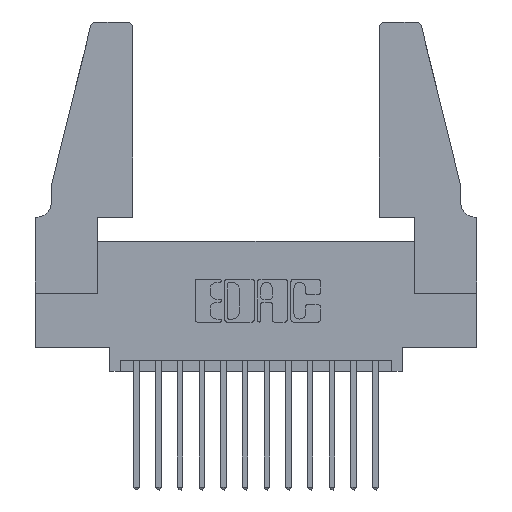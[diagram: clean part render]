
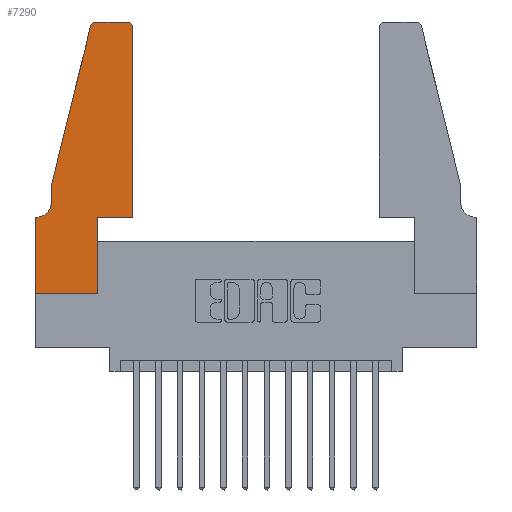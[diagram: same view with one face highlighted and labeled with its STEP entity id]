
A CAD part, top view. The second image highlights one B-rep face of the part: STEP entity #7290.
In plain terms, the highlighted planar face has unit normal (0, 0, 1).
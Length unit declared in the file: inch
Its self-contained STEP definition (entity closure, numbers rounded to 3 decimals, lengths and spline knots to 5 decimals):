
#84 = VECTOR ( 'NONE', #13092, 39.37008 ) ;
#192 = DIRECTION ( 'NONE',  ( 0., 0., 1. ) ) ;
#492 = CARTESIAN_POINT ( 'NONE',  ( 0.0755, 0.42, 0.37 ) ) ;
#546 = CARTESIAN_POINT ( 'NONE',  ( 0., 0., 0.37 ) ) ;
#605 = CARTESIAN_POINT ( 'NONE',  ( 0.0755, 0.5, 0.37 ) ) ;
#638 = AXIS2_PLACEMENT_3D ( 'NONE', #14858, #8767, #1571 ) ;
#672 = DIRECTION ( 'NONE',  ( -1., 0., 0. ) ) ;
#701 = ORIENTED_EDGE ( 'NONE', *, *, #11034, .T. ) ;
#853 = CARTESIAN_POINT ( 'NONE',  ( 0.4505, 1.22, 0.37 ) ) ;
#1107 = CARTESIAN_POINT ( 'NONE',  ( 0.4505, 0.35, 0.37 ) ) ;
#1241 = ORIENTED_EDGE ( 'NONE', *, *, #5339, .T. ) ;
#1253 = DIRECTION ( 'NONE',  ( 1., 0., 0. ) ) ;
#1389 = CARTESIAN_POINT ( 'NONE',  ( 0.25487, 1.22718, 0.37 ) ) ;
#1391 = VERTEX_POINT ( 'NONE', #3278 ) ;
#1571 = DIRECTION ( 'NONE',  ( 1., 0., 0. ) ) ;
#1697 = CARTESIAN_POINT ( 'NONE',  ( 0.0755, 0.5, 0.37 ) ) ;
#1757 = LINE ( 'NONE', #3747, #2141 ) ;
#1856 = DIRECTION ( 'NONE',  ( -1., 0., 0. ) ) ;
#1939 = EDGE_CURVE ( 'NONE', #2819, #4220, #13494, .T. ) ;
#2141 = VECTOR ( 'NONE', #10992, 39.37008 ) ;
#2243 = ORIENTED_EDGE ( 'NONE', *, *, #1939, .T. ) ;
#2408 = EDGE_CURVE ( 'NONE', #7118, #6739, #5251, .T. ) ;
#2602 = CARTESIAN_POINT ( 'NONE',  ( 0.4505, 0.35, 0.37 ) ) ;
#2819 = VERTEX_POINT ( 'NONE', #1107 ) ;
#3278 = CARTESIAN_POINT ( 'NONE',  ( 0., 0.35, 0.37 ) ) ;
#3310 = CARTESIAN_POINT ( 'NONE',  ( 0.2865, 0., 0.37 ) ) ;
#3316 = LINE ( 'NONE', #10533, #84 ) ;
#3398 = CARTESIAN_POINT ( 'NONE',  ( 0.4205, 1.25, 0.37 ) ) ;
#3677 = VERTEX_POINT ( 'NONE', #11622 ) ;
#3747 = CARTESIAN_POINT ( 'NONE',  ( 0., 0., 0.37 ) ) ;
#3849 = DIRECTION ( 'NONE',  ( -0.239, -0.971, 0. ) ) ;
#4220 = VERTEX_POINT ( 'NONE', #853 ) ;
#4300 = CARTESIAN_POINT ( 'NONE',  ( 0.0755, 0.35, 0.37 ) ) ;
#4465 = VERTEX_POINT ( 'NONE', #13793 ) ;
#5146 = EDGE_CURVE ( 'NONE', #12961, #3677, #8359, .T. ) ;
#5251 = CIRCLE ( 'NONE', #10127, 0.03 ) ;
#5339 = EDGE_CURVE ( 'NONE', #6739, #14313, #14038, .T. ) ;
#5395 = FACE_OUTER_BOUND ( 'NONE', #15324, .T. ) ;
#5674 = CARTESIAN_POINT ( 'NONE',  ( 0., 0.35, 0.37 ) ) ;
#5759 = VECTOR ( 'NONE', #14566, 39.37008 ) ;
#5849 = CARTESIAN_POINT ( 'NONE',  ( 0.0055, 0.42, 0.37 ) ) ;
#5936 = ORIENTED_EDGE ( 'NONE', *, *, #7272, .T. ) ;
#6256 = DIRECTION ( 'NONE',  ( 0., 1., 0. ) ) ;
#6335 = ORIENTED_EDGE ( 'NONE', *, *, #7974, .T. ) ;
#6739 = VERTEX_POINT ( 'NONE', #1389 ) ;
#6799 = AXIS2_PLACEMENT_3D ( 'NONE', #5674, #12247, #1253 ) ;
#6877 = ORIENTED_EDGE ( 'NONE', *, *, #12851, .T. ) ;
#6948 = CARTESIAN_POINT ( 'NONE',  ( 0.2865, 0.35, 0.37 ) ) ;
#7003 = VECTOR ( 'NONE', #6256, 39.37008 ) ;
#7049 = EDGE_CURVE ( 'NONE', #3677, #1391, #13036, .T. ) ;
#7118 = VERTEX_POINT ( 'NONE', #13945 ) ;
#7125 = ORIENTED_EDGE ( 'NONE', *, *, #9181, .T. ) ;
#7191 = VERTEX_POINT ( 'NONE', #3398 ) ;
#7272 = EDGE_CURVE ( 'NONE', #8377, #7866, #3316, .T. ) ;
#7290 = ADVANCED_FACE ( 'NONE', ( #5395 ), #13145, .T. ) ;
#7386 = CARTESIAN_POINT ( 'NONE',  ( 0.284, 1.22, 0.37 ) ) ;
#7866 = VERTEX_POINT ( 'NONE', #6948 ) ;
#7920 = ORIENTED_EDGE ( 'NONE', *, *, #7049, .T. ) ;
#7974 = EDGE_CURVE ( 'NONE', #7866, #2819, #11871, .T. ) ;
#8359 = CIRCLE ( 'NONE', #10827, 0.07 ) ;
#8377 = VERTEX_POINT ( 'NONE', #3310 ) ;
#8378 = DIRECTION ( 'NONE',  ( -1., 0., 0. ) ) ;
#8520 = VECTOR ( 'NONE', #672, 39.37008 ) ;
#8654 = DIRECTION ( 'NONE',  ( 1., 0., 0. ) ) ;
#8767 = DIRECTION ( 'NONE',  ( 0., 0., 1. ) ) ;
#9181 = EDGE_CURVE ( 'NONE', #14313, #12961, #14522, .T. ) ;
#9250 = LINE ( 'NONE', #546, #12871 ) ;
#9561 = CIRCLE ( 'NONE', #638, 0.03 ) ;
#9721 = ORIENTED_EDGE ( 'NONE', *, *, #2408, .T. ) ;
#9735 = CARTESIAN_POINT ( 'NONE',  ( 0.0755, 0.5, 0.37 ) ) ;
#10012 = ORIENTED_EDGE ( 'NONE', *, *, #5146, .T. ) ;
#10127 = AXIS2_PLACEMENT_3D ( 'NONE', #7386, #192, #8654 ) ;
#10533 = CARTESIAN_POINT ( 'NONE',  ( 0.2865, 0.35, 0.37 ) ) ;
#10610 = VECTOR ( 'NONE', #3849, 39.37008 ) ;
#10827 = AXIS2_PLACEMENT_3D ( 'NONE', #5849, #13270, #8378 ) ;
#10992 = DIRECTION ( 'NONE',  ( 1., 0., 0. ) ) ;
#11034 = EDGE_CURVE ( 'NONE', #7191, #7118, #11368, .T. ) ;
#11368 = LINE ( 'NONE', #12878, #8520 ) ;
#11458 = VECTOR ( 'NONE', #14866, 39.37008 ) ;
#11464 = DIRECTION ( 'NONE',  ( 0., -1., 0. ) ) ;
#11622 = CARTESIAN_POINT ( 'NONE',  ( 0.0055, 0.35, 0.37 ) ) ;
#11851 = ORIENTED_EDGE ( 'NONE', *, *, #14215, .T. ) ;
#11871 = LINE ( 'NONE', #14678, #5759 ) ;
#12247 = DIRECTION ( 'NONE',  ( 0., 0., 1. ) ) ;
#12851 = EDGE_CURVE ( 'NONE', #1391, #4465, #9250, .T. ) ;
#12871 = VECTOR ( 'NONE', #11464, 39.37008 ) ;
#12878 = CARTESIAN_POINT ( 'NONE',  ( 0.2605, 1.25, 0.37 ) ) ;
#12961 = VERTEX_POINT ( 'NONE', #492 ) ;
#13036 = LINE ( 'NONE', #4300, #15518 ) ;
#13092 = DIRECTION ( 'NONE',  ( 0., 1., 0. ) ) ;
#13145 = PLANE ( 'NONE',  #6799 ) ;
#13270 = DIRECTION ( 'NONE',  ( 0., 0., -1. ) ) ;
#13494 = LINE ( 'NONE', #2602, #7003 ) ;
#13793 = CARTESIAN_POINT ( 'NONE',  ( 0., 0., 0.37 ) ) ;
#13945 = CARTESIAN_POINT ( 'NONE',  ( 0.284, 1.25, 0.37 ) ) ;
#14038 = LINE ( 'NONE', #1697, #10610 ) ;
#14047 = EDGE_CURVE ( 'NONE', #4465, #8377, #1757, .T. ) ;
#14215 = EDGE_CURVE ( 'NONE', #4220, #7191, #9561, .T. ) ;
#14313 = VERTEX_POINT ( 'NONE', #605 ) ;
#14522 = LINE ( 'NONE', #9735, #11458 ) ;
#14566 = DIRECTION ( 'NONE',  ( 1., 0., 0. ) ) ;
#14678 = CARTESIAN_POINT ( 'NONE',  ( 0.4505, 0.35, 0.37 ) ) ;
#14858 = CARTESIAN_POINT ( 'NONE',  ( 0.4205, 1.22, 0.37 ) ) ;
#14866 = DIRECTION ( 'NONE',  ( 0., -1., 0. ) ) ;
#15324 = EDGE_LOOP ( 'NONE', ( #701, #9721, #1241, #7125, #10012, #7920, #6877, #15657, #5936, #6335, #2243, #11851 ) ) ;
#15518 = VECTOR ( 'NONE', #1856, 39.37008 ) ;
#15657 = ORIENTED_EDGE ( 'NONE', *, *, #14047, .T. ) ;
